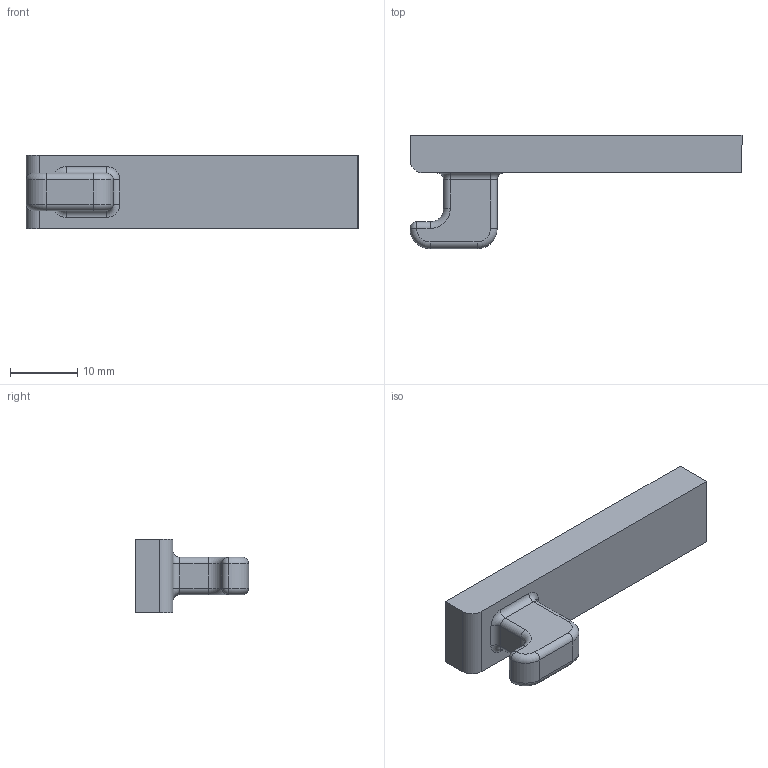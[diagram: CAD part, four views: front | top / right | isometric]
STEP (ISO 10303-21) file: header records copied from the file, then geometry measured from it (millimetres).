
FILE_DESCRIPTION((''),'2;1');
FILE_NAME('PM522GuideRod2.stp','2015-10-01T18:17:38',('JamesRPatrick'),(''),'Autodesk Inventor 2012','Autodesk Inventor 2012','');
FILE_SCHEMA(('AUTOMOTIVE_DESIGN { 1 0 10303 214 1 1 1 1 }'));
Length unit declared in the file: millimetre
Products named in the file (1): PM522GuideRod2
Bounding box: 49.5 x 16.9 x 11 mm (x, y, z)
Volume: 3630.3 mm3; surface area: 2089.1 mm2
Topology: 1 solids, 1 shells, 41 faces, 90 edges, 52 vertices
Faces by surface type: cylinder 17, plane 12, torus 10, sphere 2
Entity records: 1144 total; most frequent: DIRECTION 220, CARTESIAN_POINT 184, ORIENTED_EDGE 180, EDGE_CURVE 90, AXIS2_PLACEMENT_3D 88, VERTEX_POINT 52, CIRCLE 46, VECTOR 44
